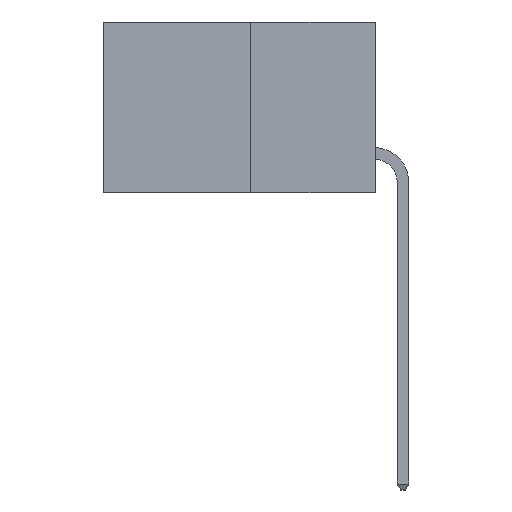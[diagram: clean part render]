
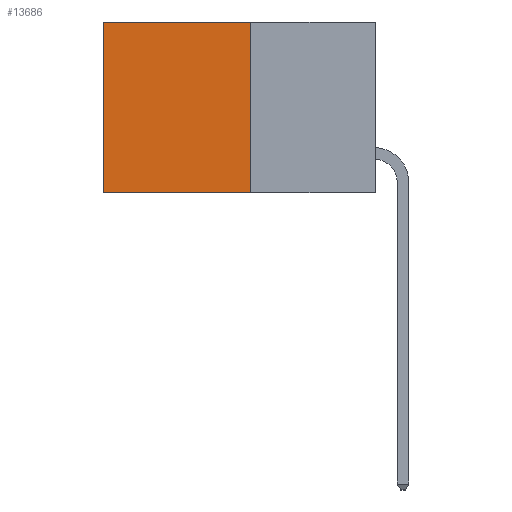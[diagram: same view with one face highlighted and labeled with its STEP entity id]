
A CAD part, left-side view. The second image highlights one B-rep face of the part: STEP entity #13686.
In plain terms, the highlighted planar face has unit normal (-1, 0, 0).
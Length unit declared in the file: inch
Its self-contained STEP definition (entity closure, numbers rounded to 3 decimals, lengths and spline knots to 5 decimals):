
#213 = LINE ( 'NONE', #1757, #9512 ) ;
#249 = CARTESIAN_POINT ( 'NONE',  ( 0.277, 0.27, 0. ) ) ;
#382 = EDGE_LOOP ( 'NONE', ( #8075, #7843, #12637, #750 ) ) ;
#461 = EDGE_CURVE ( 'NONE', #9006, #8957, #7443, .T. ) ;
#497 = LINE ( 'NONE', #9441, #10551 ) ;
#676 = LINE ( 'NONE', #3904, #14383 ) ;
#735 = CARTESIAN_POINT ( 'NONE',  ( 0.277, 0.59, 0. ) ) ;
#750 = ORIENTED_EDGE ( 'NONE', *, *, #461, .T. ) ;
#869 = CARTESIAN_POINT ( 'NONE',  ( 0.277, 0.27, 0. ) ) ;
#1396 = CARTESIAN_POINT ( 'NONE',  ( 0.277, 0.27, -0.37 ) ) ;
#1757 = CARTESIAN_POINT ( 'NONE',  ( 0.277, 0.27, -0.37 ) ) ;
#2779 = CARTESIAN_POINT ( 'NONE',  ( 0.277, 0.27, -0.37 ) ) ;
#3883 = DIRECTION ( 'NONE',  ( 0., 0., -1. ) ) ;
#3904 = CARTESIAN_POINT ( 'NONE',  ( 0.277, 0.27, -0.37 ) ) ;
#4601 = FACE_OUTER_BOUND ( 'NONE', #382, .T. ) ;
#4755 = EDGE_CURVE ( 'NONE', #8957, #13861, #497, .T. ) ;
#5895 = EDGE_CURVE ( 'NONE', #9006, #9273, #676, .T. ) ;
#6708 = DIRECTION ( 'NONE',  ( 0., 0., -1. ) ) ;
#7046 = VECTOR ( 'NONE', #13128, 39.37008 ) ;
#7443 = LINE ( 'NONE', #249, #7046 ) ;
#7843 = ORIENTED_EDGE ( 'NONE', *, *, #8817, .F. ) ;
#8075 = ORIENTED_EDGE ( 'NONE', *, *, #4755, .T. ) ;
#8817 = EDGE_CURVE ( 'NONE', #9273, #13861, #213, .T. ) ;
#8957 = VERTEX_POINT ( 'NONE', #735 ) ;
#9006 = VERTEX_POINT ( 'NONE', #869 ) ;
#9048 = DIRECTION ( 'NONE',  ( 0., 0., -1. ) ) ;
#9273 = VERTEX_POINT ( 'NONE', #1396 ) ;
#9441 = CARTESIAN_POINT ( 'NONE',  ( 0.277, 0.59, -0.37 ) ) ;
#9512 = VECTOR ( 'NONE', #9606, 39.37008 ) ;
#9606 = DIRECTION ( 'NONE',  ( 0., 1., 0. ) ) ;
#9832 = AXIS2_PLACEMENT_3D ( 'NONE', #2779, #14255, #6708 ) ;
#10551 = VECTOR ( 'NONE', #9048, 39.37008 ) ;
#12637 = ORIENTED_EDGE ( 'NONE', *, *, #5895, .F. ) ;
#13128 = DIRECTION ( 'NONE',  ( 0., 1., 0. ) ) ;
#13396 = CARTESIAN_POINT ( 'NONE',  ( 0.277, 0.59, -0.37 ) ) ;
#13686 = ADVANCED_FACE ( 'NONE', ( #4601 ), #15412, .F. ) ;
#13861 = VERTEX_POINT ( 'NONE', #13396 ) ;
#14255 = DIRECTION ( 'NONE',  ( 1., 0., 0. ) ) ;
#14383 = VECTOR ( 'NONE', #3883, 39.37008 ) ;
#15412 = PLANE ( 'NONE',  #9832 ) ;
